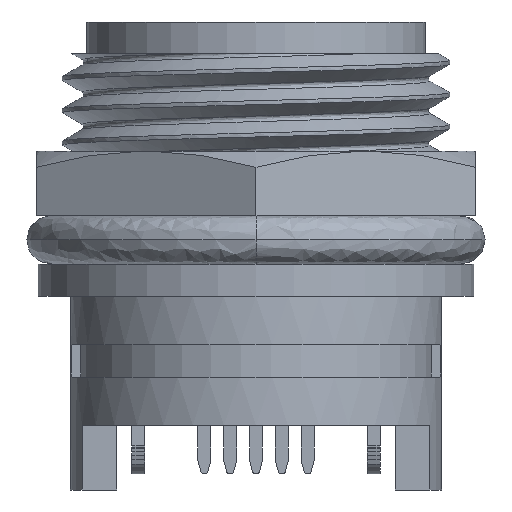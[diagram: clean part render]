
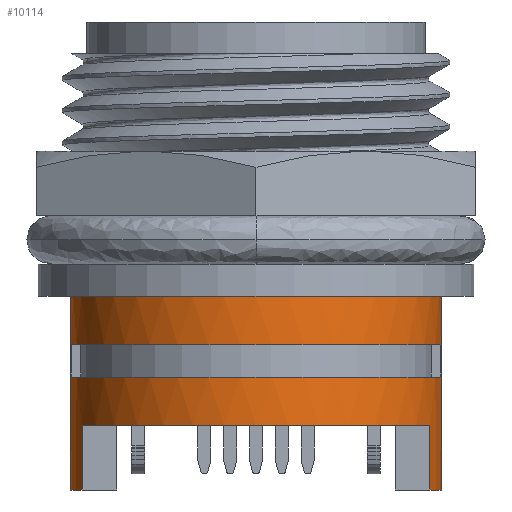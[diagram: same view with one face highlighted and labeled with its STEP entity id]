
A CAD part, front view. The second image highlights one B-rep face of the part: STEP entity #10114.
In plain terms, the highlighted cylindrical face has radius 5.75 mm (diameter 11.5 mm), a partial arc.
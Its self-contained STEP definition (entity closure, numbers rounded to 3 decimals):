
#113 = DIRECTION ( 'NONE',  ( -1., 0., 0. ) ) ;
#270 = CARTESIAN_POINT ( 'NONE',  ( -5.728, -0.5, -10. ) ) ;
#282 = CARTESIAN_POINT ( 'NONE',  ( 0., 0., -14.5 ) ) ;
#315 = AXIS2_PLACEMENT_3D ( 'NONE', #34554, #31898, #7530 ) ;
#389 = VERTEX_POINT ( 'NONE', #3255 ) ;
#872 = CARTESIAN_POINT ( 'NONE',  ( 5.391, -2., -14.5 ) ) ;
#1028 = CARTESIAN_POINT ( 'NONE',  ( -5.75, 0., -14.5 ) ) ;
#1131 = AXIS2_PLACEMENT_3D ( 'NONE', #282, #16871, #14022 ) ;
#1319 = DIRECTION ( 'NONE',  ( 0., 0., 1. ) ) ;
#2715 = ORIENTED_EDGE ( 'NONE', *, *, #6163, .T. ) ;
#2959 = DIRECTION ( 'NONE',  ( 0., 0., -1. ) ) ;
#3255 = CARTESIAN_POINT ( 'NONE',  ( -5.728, -0.5, -11. ) ) ;
#3866 = ORIENTED_EDGE ( 'NONE', *, *, #32271, .F. ) ;
#4533 = CARTESIAN_POINT ( 'NONE',  ( -5.728, -0.5, -8.38 ) ) ;
#4704 = ORIENTED_EDGE ( 'NONE', *, *, #21615, .T. ) ;
#4803 = LINE ( 'NONE', #29504, #29674 ) ;
#4977 = DIRECTION ( 'NONE',  ( -1., 0., 0. ) ) ;
#5020 = CYLINDRICAL_SURFACE ( 'NONE', #315, 5.75 ) ;
#5186 = DIRECTION ( 'NONE',  ( -1., 0., 0. ) ) ;
#5211 = AXIS2_PLACEMENT_3D ( 'NONE', #13673, #24521, #113 ) ;
#5345 = EDGE_CURVE ( 'NONE', #20467, #10321, #24452, .T. ) ;
#5616 = AXIS2_PLACEMENT_3D ( 'NONE', #30368, #22206, #25368 ) ;
#6089 = VECTOR ( 'NONE', #2959, 1000. ) ;
#6163 = EDGE_CURVE ( 'NONE', #16043, #25564, #4803, .T. ) ;
#6318 = VERTEX_POINT ( 'NONE', #27192 ) ;
#7530 = DIRECTION ( 'NONE',  ( -1., 0., 0. ) ) ;
#7690 = FACE_BOUND ( 'NONE', #35196, .T. ) ;
#8189 = ORIENTED_EDGE ( 'NONE', *, *, #24717, .T. ) ;
#8261 = CARTESIAN_POINT ( 'NONE',  ( 5.391, -2., -8.38 ) ) ;
#8572 = ORIENTED_EDGE ( 'NONE', *, *, #28398, .T. ) ;
#8705 = VERTEX_POINT ( 'NONE', #270 ) ;
#8733 = DIRECTION ( 'NONE',  ( 0., 0., 1. ) ) ;
#9590 = CIRCLE ( 'NONE', #5616, 5.75 ) ;
#10114 = ADVANCED_FACE ( 'NONE', ( #12868, #7690 ), #5020, .T. ) ;
#10292 = VERTEX_POINT ( 'NONE', #30279 ) ;
#10321 = VERTEX_POINT ( 'NONE', #872 ) ;
#10905 = CIRCLE ( 'NONE', #18328, 5.75 ) ;
#11265 = CARTESIAN_POINT ( 'NONE',  ( 5.75, 0., -8.38 ) ) ;
#11467 = VECTOR ( 'NONE', #29761, 1000. ) ;
#12157 = CARTESIAN_POINT ( 'NONE',  ( 5.75, 0., -8.5 ) ) ;
#12868 = FACE_OUTER_BOUND ( 'NONE', #33155, .T. ) ;
#13093 = LINE ( 'NONE', #31601, #29000 ) ;
#13666 = CARTESIAN_POINT ( 'NONE',  ( -5.75, 0., -8.38 ) ) ;
#13673 = CARTESIAN_POINT ( 'NONE',  ( 0., 0., -8.5 ) ) ;
#13908 = ORIENTED_EDGE ( 'NONE', *, *, #31370, .T. ) ;
#14022 = DIRECTION ( 'NONE',  ( -1., 0., 0. ) ) ;
#14409 = DIRECTION ( 'NONE',  ( 0., 0., 1. ) ) ;
#15754 = EDGE_CURVE ( 'NONE', #8705, #26964, #20299, .T. ) ;
#16043 = VERTEX_POINT ( 'NONE', #18490 ) ;
#16665 = VERTEX_POINT ( 'NONE', #12157 ) ;
#16871 = DIRECTION ( 'NONE',  ( 0., 0., 1. ) ) ;
#18295 = CARTESIAN_POINT ( 'NONE',  ( 5.75, 0., -14.5 ) ) ;
#18328 = AXIS2_PLACEMENT_3D ( 'NONE', #24762, #8733, #5186 ) ;
#18453 = EDGE_CURVE ( 'NONE', #16665, #6318, #30225, .T. ) ;
#18490 = CARTESIAN_POINT ( 'NONE',  ( -5.391, -2., -14.5 ) ) ;
#18563 = AXIS2_PLACEMENT_3D ( 'NONE', #19418, #14409, #30049 ) ;
#18939 = LINE ( 'NONE', #11265, #11467 ) ;
#19418 = CARTESIAN_POINT ( 'NONE',  ( 0., 0., -10. ) ) ;
#20299 = CIRCLE ( 'NONE', #18563, 5.75 ) ;
#20458 = ORIENTED_EDGE ( 'NONE', *, *, #15754, .T. ) ;
#20467 = VERTEX_POINT ( 'NONE', #24649 ) ;
#20727 = ORIENTED_EDGE ( 'NONE', *, *, #30337, .T. ) ;
#21083 = CIRCLE ( 'NONE', #1131, 5.75 ) ;
#21615 = EDGE_CURVE ( 'NONE', #6318, #33686, #24700, .T. ) ;
#22206 = DIRECTION ( 'NONE',  ( 0., 0., 1. ) ) ;
#23153 = EDGE_CURVE ( 'NONE', #25564, #20467, #9590, .T. ) ;
#23328 = VECTOR ( 'NONE', #29788, 1000. ) ;
#23333 = ORIENTED_EDGE ( 'NONE', *, *, #5345, .T. ) ;
#23616 = CARTESIAN_POINT ( 'NONE',  ( -5.391, -2., -12.5 ) ) ;
#23950 = DIRECTION ( 'NONE',  ( 0., 0., -1. ) ) ;
#24452 = LINE ( 'NONE', #8261, #23328 ) ;
#24521 = DIRECTION ( 'NONE',  ( 0., 0., -1. ) ) ;
#24649 = CARTESIAN_POINT ( 'NONE',  ( 5.391, -2., -12.5 ) ) ;
#24700 = LINE ( 'NONE', #13666, #6089 ) ;
#24717 = EDGE_CURVE ( 'NONE', #10292, #389, #31806, .T. ) ;
#24762 = CARTESIAN_POINT ( 'NONE',  ( 0., 0., -14.5 ) ) ;
#25368 = DIRECTION ( 'NONE',  ( -1., 0., 0. ) ) ;
#25564 = VERTEX_POINT ( 'NONE', #23616 ) ;
#26118 = AXIS2_PLACEMENT_3D ( 'NONE', #29519, #31849, #4977 ) ;
#26964 = VERTEX_POINT ( 'NONE', #30079 ) ;
#27192 = CARTESIAN_POINT ( 'NONE',  ( -5.75, 0., -8.5 ) ) ;
#27318 = ORIENTED_EDGE ( 'NONE', *, *, #18453, .T. ) ;
#27557 = VERTEX_POINT ( 'NONE', #18295 ) ;
#28115 = EDGE_CURVE ( 'NONE', #10321, #27557, #21083, .T. ) ;
#28398 = EDGE_CURVE ( 'NONE', #26964, #10292, #13093, .T. ) ;
#28742 = LINE ( 'NONE', #4533, #30883 ) ;
#29000 = VECTOR ( 'NONE', #23950, 1000. ) ;
#29504 = CARTESIAN_POINT ( 'NONE',  ( -5.391, -2., -8.38 ) ) ;
#29519 = CARTESIAN_POINT ( 'NONE',  ( 0., 0., -11. ) ) ;
#29674 = VECTOR ( 'NONE', #34674, 1000. ) ;
#29761 = DIRECTION ( 'NONE',  ( 0., 0., -1. ) ) ;
#29788 = DIRECTION ( 'NONE',  ( 0., 0., -1. ) ) ;
#30049 = DIRECTION ( 'NONE',  ( -1., 0., 0. ) ) ;
#30079 = CARTESIAN_POINT ( 'NONE',  ( 5.728, -0.5, -10. ) ) ;
#30225 = CIRCLE ( 'NONE', #5211, 5.75 ) ;
#30277 = ORIENTED_EDGE ( 'NONE', *, *, #28115, .T. ) ;
#30279 = CARTESIAN_POINT ( 'NONE',  ( 5.728, -0.5, -11. ) ) ;
#30337 = EDGE_CURVE ( 'NONE', #33686, #16043, #10905, .T. ) ;
#30368 = CARTESIAN_POINT ( 'NONE',  ( 0., 0., -12.5 ) ) ;
#30883 = VECTOR ( 'NONE', #1319, 1000. ) ;
#31128 = ORIENTED_EDGE ( 'NONE', *, *, #23153, .T. ) ;
#31370 = EDGE_CURVE ( 'NONE', #389, #8705, #28742, .T. ) ;
#31601 = CARTESIAN_POINT ( 'NONE',  ( 5.728, -0.5, -8.38 ) ) ;
#31806 = CIRCLE ( 'NONE', #26118, 5.75 ) ;
#31849 = DIRECTION ( 'NONE',  ( 0., 0., -1. ) ) ;
#31898 = DIRECTION ( 'NONE',  ( 0., 0., -1. ) ) ;
#32271 = EDGE_CURVE ( 'NONE', #16665, #27557, #18939, .T. ) ;
#33155 = EDGE_LOOP ( 'NONE', ( #3866, #27318, #4704, #20727, #2715, #31128, #23333, #30277 ) ) ;
#33686 = VERTEX_POINT ( 'NONE', #1028 ) ;
#34554 = CARTESIAN_POINT ( 'NONE',  ( 0., 0., -8.38 ) ) ;
#34674 = DIRECTION ( 'NONE',  ( 0., 0., 1. ) ) ;
#35196 = EDGE_LOOP ( 'NONE', ( #8189, #13908, #20458, #8572 ) ) ;
